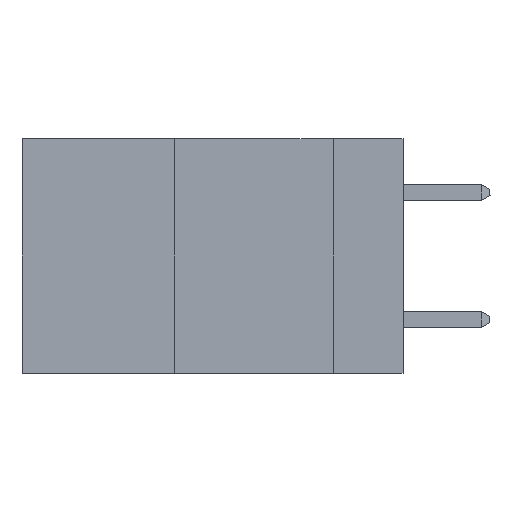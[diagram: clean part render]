
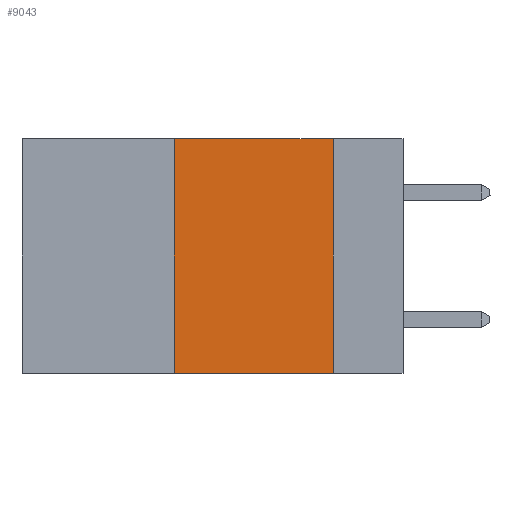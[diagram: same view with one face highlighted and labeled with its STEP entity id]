
A CAD part, left-side view. The second image highlights one B-rep face of the part: STEP entity #9043.
In plain terms, the highlighted planar face has unit normal (-1, 0, 0).
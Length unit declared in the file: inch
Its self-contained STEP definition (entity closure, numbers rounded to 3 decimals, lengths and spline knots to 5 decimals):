
#2842 = FACE_OUTER_BOUND ( 'NONE', #9032, .T. ) ;
#3005 = EDGE_CURVE ( 'NONE', #22822, #7725, #33419, .T. ) ;
#3129 = DIRECTION ( 'NONE',  ( 0., 0., -1. ) ) ;
#3173 = VECTOR ( 'NONE', #22215, 39.37008 ) ;
#6883 = VERTEX_POINT ( 'NONE', #18933 ) ;
#7725 = VERTEX_POINT ( 'NONE', #24117 ) ;
#8605 = LINE ( 'NONE', #9003, #16100 ) ;
#8664 = VECTOR ( 'NONE', #38918, 39.37008 ) ;
#8907 = PLANE ( 'NONE',  #27889 ) ;
#9003 = CARTESIAN_POINT ( 'NONE',  ( 0., 0.11, 0. ) ) ;
#9032 = EDGE_LOOP ( 'NONE', ( #13302, #21371, #14034, #24220 ) ) ;
#9043 = ADVANCED_FACE ( 'NONE', ( #2842 ), #8907, .F. ) ;
#9863 = LINE ( 'NONE', #21809, #3173 ) ;
#11238 = CARTESIAN_POINT ( 'NONE',  ( 0., 0.36, 0. ) ) ;
#11428 = LINE ( 'NONE', #11238, #34740 ) ;
#11625 = VERTEX_POINT ( 'NONE', #14379 ) ;
#11638 = DIRECTION ( 'NONE',  ( 0., 0., 1. ) ) ;
#13302 = ORIENTED_EDGE ( 'NONE', *, *, #36822, .F. ) ;
#14034 = ORIENTED_EDGE ( 'NONE', *, *, #20819, .F. ) ;
#14379 = CARTESIAN_POINT ( 'NONE',  ( 0., 0.36, -0.37 ) ) ;
#15180 = DIRECTION ( 'NONE',  ( 0., 0., -1. ) ) ;
#16100 = VECTOR ( 'NONE', #3129, 39.37008 ) ;
#18235 = DIRECTION ( 'NONE',  ( 1., 0., 0. ) ) ;
#18933 = CARTESIAN_POINT ( 'NONE',  ( 0., 0.11, -0.37 ) ) ;
#20819 = EDGE_CURVE ( 'NONE', #11625, #22822, #11428, .T. ) ;
#21371 = ORIENTED_EDGE ( 'NONE', *, *, #3005, .F. ) ;
#21809 = CARTESIAN_POINT ( 'NONE',  ( 0., 0.6, -0.37 ) ) ;
#22215 = DIRECTION ( 'NONE',  ( 0., -1., 0. ) ) ;
#22822 = VERTEX_POINT ( 'NONE', #24639 ) ;
#24117 = CARTESIAN_POINT ( 'NONE',  ( 0., 0.11, 0. ) ) ;
#24220 = ORIENTED_EDGE ( 'NONE', *, *, #36578, .T. ) ;
#24639 = CARTESIAN_POINT ( 'NONE',  ( 0., 0.36, 0. ) ) ;
#26738 = CARTESIAN_POINT ( 'NONE',  ( 0., 0.6, 0. ) ) ;
#27889 = AXIS2_PLACEMENT_3D ( 'NONE', #30811, #18235, #15180 ) ;
#30811 = CARTESIAN_POINT ( 'NONE',  ( 0., 0.6, 0. ) ) ;
#33419 = LINE ( 'NONE', #26738, #8664 ) ;
#34740 = VECTOR ( 'NONE', #11638, 39.37008 ) ;
#36578 = EDGE_CURVE ( 'NONE', #11625, #6883, #9863, .T. ) ;
#36822 = EDGE_CURVE ( 'NONE', #7725, #6883, #8605, .T. ) ;
#38918 = DIRECTION ( 'NONE',  ( 0., -1., 0. ) ) ;
